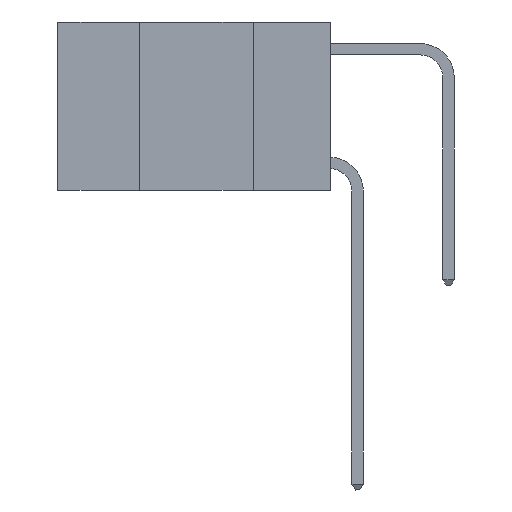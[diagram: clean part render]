
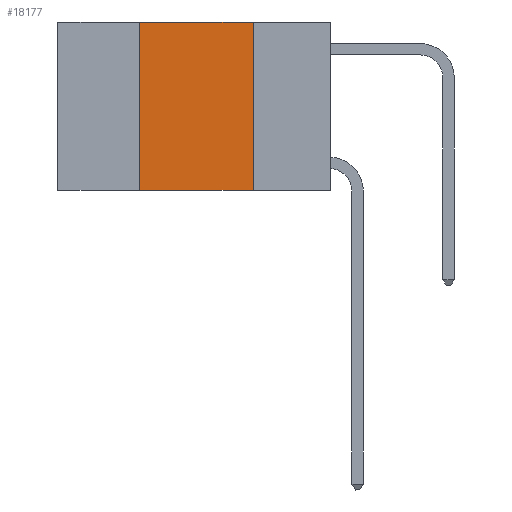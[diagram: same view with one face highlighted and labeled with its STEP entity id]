
A CAD part, left-side view. The second image highlights one B-rep face of the part: STEP entity #18177.
In plain terms, the highlighted planar face has unit normal (-1, 0, 0).
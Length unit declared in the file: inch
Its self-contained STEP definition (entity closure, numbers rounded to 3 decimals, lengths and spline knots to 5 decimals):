
#512 = ORIENTED_EDGE ( 'NONE', *, *, #2792, .F. ) ;
#722 = EDGE_CURVE ( 'NONE', #19732, #2004, #2926, .T. ) ;
#1540 = ORIENTED_EDGE ( 'NONE', *, *, #14346, .F. ) ;
#2004 = VERTEX_POINT ( 'NONE', #11379 ) ;
#2225 = LINE ( 'NONE', #14225, #18500 ) ;
#2792 = EDGE_CURVE ( 'NONE', #19732, #14435, #2225, .T. ) ;
#2926 = LINE ( 'NONE', #19768, #12160 ) ;
#2966 = CARTESIAN_POINT ( 'NONE',  ( 0., 0.42, 0. ) ) ;
#3144 = VECTOR ( 'NONE', #8611, 39.37008 ) ;
#3455 = ORIENTED_EDGE ( 'NONE', *, *, #722, .T. ) ;
#3706 = AXIS2_PLACEMENT_3D ( 'NONE', #14561, #9924, #11346 ) ;
#4163 = DIRECTION ( 'NONE',  ( 0., -1., 0. ) ) ;
#4908 = ORIENTED_EDGE ( 'NONE', *, *, #10500, .F. ) ;
#6734 = VECTOR ( 'NONE', #9876, 39.37008 ) ;
#6757 = CARTESIAN_POINT ( 'NONE',  ( 0., 0.6, 0. ) ) ;
#8611 = DIRECTION ( 'NONE',  ( 0., 0., -1. ) ) ;
#9344 = CARTESIAN_POINT ( 'NONE',  ( 0., 0.42, -0.37 ) ) ;
#9605 = EDGE_LOOP ( 'NONE', ( #1540, #4908, #512, #3455 ) ) ;
#9824 = FACE_OUTER_BOUND ( 'NONE', #9605, .T. ) ;
#9876 = DIRECTION ( 'NONE',  ( 0., -1., 0. ) ) ;
#9924 = DIRECTION ( 'NONE',  ( 1., 0., 0. ) ) ;
#10500 = EDGE_CURVE ( 'NONE', #14435, #19107, #13006, .T. ) ;
#11346 = DIRECTION ( 'NONE',  ( 0., 0., -1. ) ) ;
#11379 = CARTESIAN_POINT ( 'NONE',  ( 0., 0.17, -0.37 ) ) ;
#12160 = VECTOR ( 'NONE', #4163, 39.37008 ) ;
#12245 = DIRECTION ( 'NONE',  ( 0., 0., 1. ) ) ;
#13006 = LINE ( 'NONE', #6757, #6734 ) ;
#13359 = CARTESIAN_POINT ( 'NONE',  ( 0., 0.17, 0. ) ) ;
#14225 = CARTESIAN_POINT ( 'NONE',  ( 0., 0.42, 0. ) ) ;
#14346 = EDGE_CURVE ( 'NONE', #19107, #2004, #19432, .T. ) ;
#14435 = VERTEX_POINT ( 'NONE', #2966 ) ;
#14561 = CARTESIAN_POINT ( 'NONE',  ( 0., 0.6, 0. ) ) ;
#14761 = PLANE ( 'NONE',  #3706 ) ;
#18063 = CARTESIAN_POINT ( 'NONE',  ( 0., 0.17, 0. ) ) ;
#18177 = ADVANCED_FACE ( 'NONE', ( #9824 ), #14761, .F. ) ;
#18500 = VECTOR ( 'NONE', #12245, 39.37008 ) ;
#19107 = VERTEX_POINT ( 'NONE', #18063 ) ;
#19432 = LINE ( 'NONE', #13359, #3144 ) ;
#19732 = VERTEX_POINT ( 'NONE', #9344 ) ;
#19768 = CARTESIAN_POINT ( 'NONE',  ( 0., 0.6, -0.37 ) ) ;
